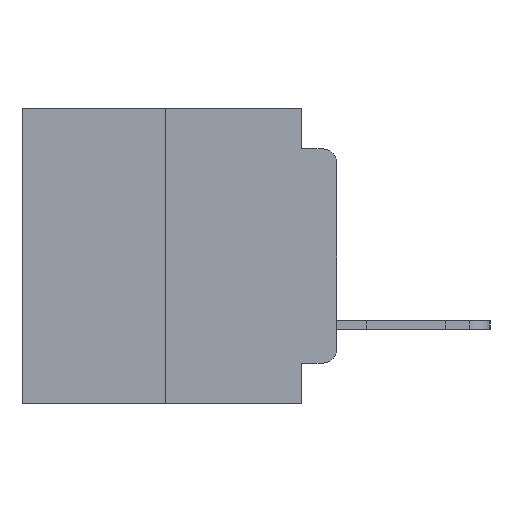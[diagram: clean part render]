
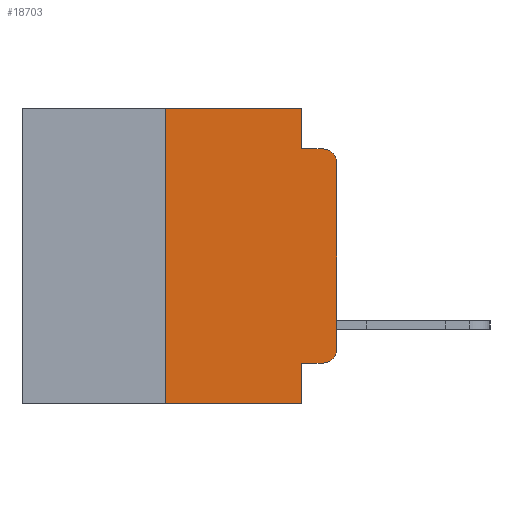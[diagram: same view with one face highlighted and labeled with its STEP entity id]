
A CAD part, left-side view. The second image highlights one B-rep face of the part: STEP entity #18703.
In plain terms, the highlighted planar face has unit normal (-1, 0, 0).
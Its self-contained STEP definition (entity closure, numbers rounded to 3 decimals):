
#310 = DIRECTION ( 'NONE',  ( 0., -1., 0. ) ) ;
#405 = DIRECTION ( 'NONE',  ( 1., 0., 0. ) ) ;
#463 = VERTEX_POINT ( 'NONE', #11232 ) ;
#495 = PLANE ( 'NONE',  #2187 ) ;
#505 = LINE ( 'NONE', #16287, #23805 ) ;
#1168 = LINE ( 'NONE', #18916, #3222 ) ;
#1407 = CARTESIAN_POINT ( 'NONE',  ( -75.603, 0., 5.486 ) ) ;
#2109 = VERTEX_POINT ( 'NONE', #26892 ) ;
#2187 = AXIS2_PLACEMENT_3D ( 'NONE', #2721, #405, #22142 ) ;
#2237 = DIRECTION ( 'NONE',  ( 0., 0., -1. ) ) ;
#2241 = VERTEX_POINT ( 'NONE', #9673 ) ;
#2345 = CARTESIAN_POINT ( 'NONE',  ( -75.603, 1.295, -3.975 ) ) ;
#2457 = DIRECTION ( 'NONE',  ( 0., 0., 1. ) ) ;
#2516 = VERTEX_POINT ( 'NONE', #4161 ) ;
#2721 = CARTESIAN_POINT ( 'NONE',  ( -75.603, 11.684, 5.486 ) ) ;
#2927 = FACE_OUTER_BOUND ( 'NONE', #12769, .T. ) ;
#3222 = VECTOR ( 'NONE', #5820, 1000. ) ;
#3506 = DIRECTION ( 'NONE',  ( 0., 0., 1. ) ) ;
#3954 = LINE ( 'NONE', #2345, #26954 ) ;
#4161 = CARTESIAN_POINT ( 'NONE',  ( -75.603, 1.295, 3.975 ) ) ;
#4343 = AXIS2_PLACEMENT_3D ( 'NONE', #11439, #9216, #17902 ) ;
#4883 = EDGE_CURVE ( 'NONE', #2516, #5753, #25600, .T. ) ;
#4913 = CARTESIAN_POINT ( 'NONE',  ( -75.603, 1.295, 3.975 ) ) ;
#5354 = EDGE_CURVE ( 'NONE', #13569, #2241, #9842, .T. ) ;
#5368 = DIRECTION ( 'NONE',  ( 0., -1., 0. ) ) ;
#5753 = VERTEX_POINT ( 'NONE', #12175 ) ;
#5820 = DIRECTION ( 'NONE',  ( 0., -1., 0. ) ) ;
#5949 = VERTEX_POINT ( 'NONE', #17392 ) ;
#6877 = AXIS2_PLACEMENT_3D ( 'NONE', #17803, #26527, #15424 ) ;
#6989 = CARTESIAN_POINT ( 'NONE',  ( -75.603, 1.295, 5.486 ) ) ;
#7080 = EDGE_CURVE ( 'NONE', #22825, #463, #26402, .T. ) ;
#8676 = CIRCLE ( 'NONE', #4343, 0.508 ) ;
#8996 = ORIENTED_EDGE ( 'NONE', *, *, #22695, .F. ) ;
#9216 = DIRECTION ( 'NONE',  ( -1., 0., 0. ) ) ;
#9387 = VERTEX_POINT ( 'NONE', #6989 ) ;
#9673 = CARTESIAN_POINT ( 'NONE',  ( -75.603, 0., -3.467 ) ) ;
#9688 = EDGE_CURVE ( 'NONE', #2241, #5949, #18329, .T. ) ;
#9842 = CIRCLE ( 'NONE', #6877, 0.508 ) ;
#10665 = EDGE_CURVE ( 'NONE', #463, #9387, #505, .T. ) ;
#10701 = CARTESIAN_POINT ( 'NONE',  ( -75.603, 1.295, 0. ) ) ;
#11232 = CARTESIAN_POINT ( 'NONE',  ( -75.603, 6.35, 5.486 ) ) ;
#11439 = CARTESIAN_POINT ( 'NONE',  ( -75.603, 0.508, 3.467 ) ) ;
#11462 = DIRECTION ( 'NONE',  ( 0., -1., 0. ) ) ;
#11493 = EDGE_CURVE ( 'NONE', #22825, #2109, #1168, .T. ) ;
#12175 = CARTESIAN_POINT ( 'NONE',  ( -75.603, 0.508, 3.975 ) ) ;
#12281 = VECTOR ( 'NONE', #2457, 1000. ) ;
#12769 = EDGE_LOOP ( 'NONE', ( #20825, #18192, #19085, #20600, #19887, #8996, #18060, #17852, #13634, #18597 ) ) ;
#13569 = VERTEX_POINT ( 'NONE', #24299 ) ;
#13634 = ORIENTED_EDGE ( 'NONE', *, *, #11493, .T. ) ;
#15424 = DIRECTION ( 'NONE',  ( 0., 0., -1. ) ) ;
#15599 = CARTESIAN_POINT ( 'NONE',  ( -75.603, 6.35, -5.486 ) ) ;
#16287 = CARTESIAN_POINT ( 'NONE',  ( -75.603, 11.684, 5.486 ) ) ;
#17392 = CARTESIAN_POINT ( 'NONE',  ( -75.603, 0., 3.467 ) ) ;
#17803 = CARTESIAN_POINT ( 'NONE',  ( -75.603, 0.508, -3.467 ) ) ;
#17852 = ORIENTED_EDGE ( 'NONE', *, *, #7080, .F. ) ;
#17902 = DIRECTION ( 'NONE',  ( 0., 0., -1. ) ) ;
#18060 = ORIENTED_EDGE ( 'NONE', *, *, #10665, .F. ) ;
#18192 = ORIENTED_EDGE ( 'NONE', *, *, #5354, .T. ) ;
#18329 = LINE ( 'NONE', #1407, #25542 ) ;
#18487 = VERTEX_POINT ( 'NONE', #25977 ) ;
#18597 = ORIENTED_EDGE ( 'NONE', *, *, #24807, .F. ) ;
#18703 = ADVANCED_FACE ( 'NONE', ( #2927 ), #495, .F. ) ;
#18916 = CARTESIAN_POINT ( 'NONE',  ( -75.603, 11.684, -5.486 ) ) ;
#19085 = ORIENTED_EDGE ( 'NONE', *, *, #9688, .T. ) ;
#19433 = VECTOR ( 'NONE', #11462, 1000. ) ;
#19887 = ORIENTED_EDGE ( 'NONE', *, *, #4883, .F. ) ;
#20503 = VECTOR ( 'NONE', #24303, 1000. ) ;
#20600 = ORIENTED_EDGE ( 'NONE', *, *, #27117, .T. ) ;
#20825 = ORIENTED_EDGE ( 'NONE', *, *, #24051, .T. ) ;
#21076 = VECTOR ( 'NONE', #2237, 1000. ) ;
#21740 = LINE ( 'NONE', #10701, #21076 ) ;
#22142 = DIRECTION ( 'NONE',  ( 0., 0., -1. ) ) ;
#22552 = LINE ( 'NONE', #26519, #20503 ) ;
#22695 = EDGE_CURVE ( 'NONE', #9387, #2516, #22552, .T. ) ;
#22825 = VERTEX_POINT ( 'NONE', #15599 ) ;
#23805 = VECTOR ( 'NONE', #5368, 1000. ) ;
#24051 = EDGE_CURVE ( 'NONE', #18487, #13569, #3954, .T. ) ;
#24087 = CARTESIAN_POINT ( 'NONE',  ( -75.603, 6.35, -5.486 ) ) ;
#24299 = CARTESIAN_POINT ( 'NONE',  ( -75.603, 0.508, -3.975 ) ) ;
#24303 = DIRECTION ( 'NONE',  ( 0., 0., -1. ) ) ;
#24807 = EDGE_CURVE ( 'NONE', #18487, #2109, #21740, .T. ) ;
#25542 = VECTOR ( 'NONE', #3506, 1000. ) ;
#25600 = LINE ( 'NONE', #4913, #19433 ) ;
#25977 = CARTESIAN_POINT ( 'NONE',  ( -75.603, 1.295, -3.975 ) ) ;
#26402 = LINE ( 'NONE', #24087, #12281 ) ;
#26519 = CARTESIAN_POINT ( 'NONE',  ( -75.603, 1.295, 0. ) ) ;
#26527 = DIRECTION ( 'NONE',  ( -1., 0., 0. ) ) ;
#26892 = CARTESIAN_POINT ( 'NONE',  ( -75.603, 1.295, -5.486 ) ) ;
#26954 = VECTOR ( 'NONE', #310, 1000. ) ;
#27117 = EDGE_CURVE ( 'NONE', #5949, #5753, #8676, .T. ) ;
